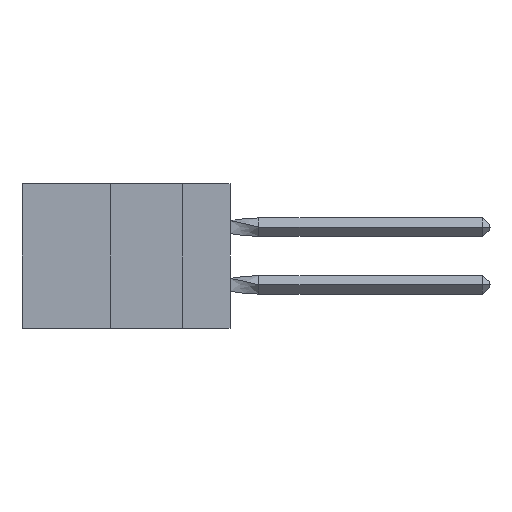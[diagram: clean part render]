
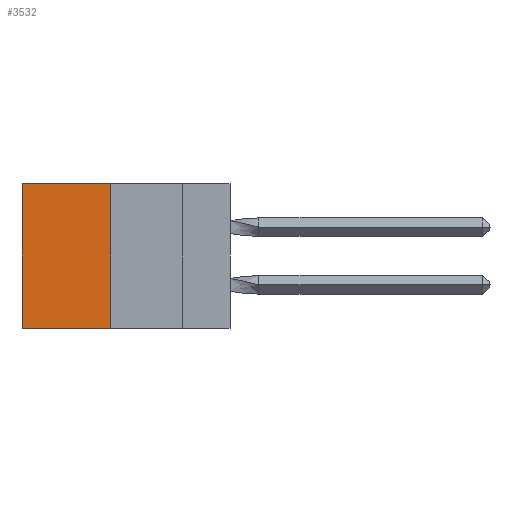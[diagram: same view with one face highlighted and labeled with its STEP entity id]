
A CAD part, left-side view. The second image highlights one B-rep face of the part: STEP entity #3532.
In plain terms, the highlighted planar face has unit normal (-1, 0, 0).
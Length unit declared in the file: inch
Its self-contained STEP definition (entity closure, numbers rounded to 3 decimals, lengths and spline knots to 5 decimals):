
#846 = VECTOR ( 'NONE', #19237, 39.37008 ) ;
#959 = ORIENTED_EDGE ( 'NONE', *, *, #5308, .T. ) ;
#1018 = DIRECTION ( 'NONE',  ( 0., 0., -1. ) ) ;
#1153 = CARTESIAN_POINT ( 'NONE',  ( 0.305, 0.413, 0. ) ) ;
#1361 = VERTEX_POINT ( 'NONE', #1153 ) ;
#1688 = LINE ( 'NONE', #11185, #38397 ) ;
#1907 = CARTESIAN_POINT ( 'NONE',  ( 0.305, 0.72, -0.5 ) ) ;
#3532 = ADVANCED_FACE ( 'NONE', ( #35233 ), #29946, .F. ) ;
#4514 = CARTESIAN_POINT ( 'NONE',  ( 0.305, 0.413, -0.5 ) ) ;
#5308 = EDGE_CURVE ( 'NONE', #1361, #35424, #6231, .T. ) ;
#5346 = ORIENTED_EDGE ( 'NONE', *, *, #27198, .T. ) ;
#6231 = LINE ( 'NONE', #18391, #14658 ) ;
#7503 = DIRECTION ( 'NONE',  ( 1., 0., 0. ) ) ;
#8130 = CARTESIAN_POINT ( 'NONE',  ( 0.305, 0.72, 0. ) ) ;
#8789 = VERTEX_POINT ( 'NONE', #4514 ) ;
#11185 = CARTESIAN_POINT ( 'NONE',  ( 0.305, 0.413, -0.5 ) ) ;
#11622 = CARTESIAN_POINT ( 'NONE',  ( 0.305, 0.72, -0.5 ) ) ;
#11857 = AXIS2_PLACEMENT_3D ( 'NONE', #35674, #7503, #1018 ) ;
#14106 = EDGE_CURVE ( 'NONE', #1361, #8789, #32076, .T. ) ;
#14241 = ORIENTED_EDGE ( 'NONE', *, *, #14106, .F. ) ;
#14658 = VECTOR ( 'NONE', #24845, 39.37008 ) ;
#15289 = DIRECTION ( 'NONE',  ( 0., 0., -1. ) ) ;
#18391 = CARTESIAN_POINT ( 'NONE',  ( 0.305, 0.413, 0. ) ) ;
#19237 = DIRECTION ( 'NONE',  ( 0., 0., -1. ) ) ;
#23601 = EDGE_CURVE ( 'NONE', #8789, #36707, #1688, .T. ) ;
#23933 = VECTOR ( 'NONE', #15289, 39.37008 ) ;
#24845 = DIRECTION ( 'NONE',  ( 0., 1., 0. ) ) ;
#27198 = EDGE_CURVE ( 'NONE', #35424, #36707, #31872, .T. ) ;
#28643 = CARTESIAN_POINT ( 'NONE',  ( 0.305, 0.413, -0.5 ) ) ;
#29946 = PLANE ( 'NONE',  #11857 ) ;
#31872 = LINE ( 'NONE', #1907, #23933 ) ;
#32076 = LINE ( 'NONE', #28643, #846 ) ;
#33760 = DIRECTION ( 'NONE',  ( 0., 1., 0. ) ) ;
#34644 = ORIENTED_EDGE ( 'NONE', *, *, #23601, .F. ) ;
#35233 = FACE_OUTER_BOUND ( 'NONE', #35977, .T. ) ;
#35424 = VERTEX_POINT ( 'NONE', #8130 ) ;
#35674 = CARTESIAN_POINT ( 'NONE',  ( 0.305, 0.413, -0.5 ) ) ;
#35977 = EDGE_LOOP ( 'NONE', ( #5346, #34644, #14241, #959 ) ) ;
#36707 = VERTEX_POINT ( 'NONE', #11622 ) ;
#38397 = VECTOR ( 'NONE', #33760, 39.37008 ) ;
